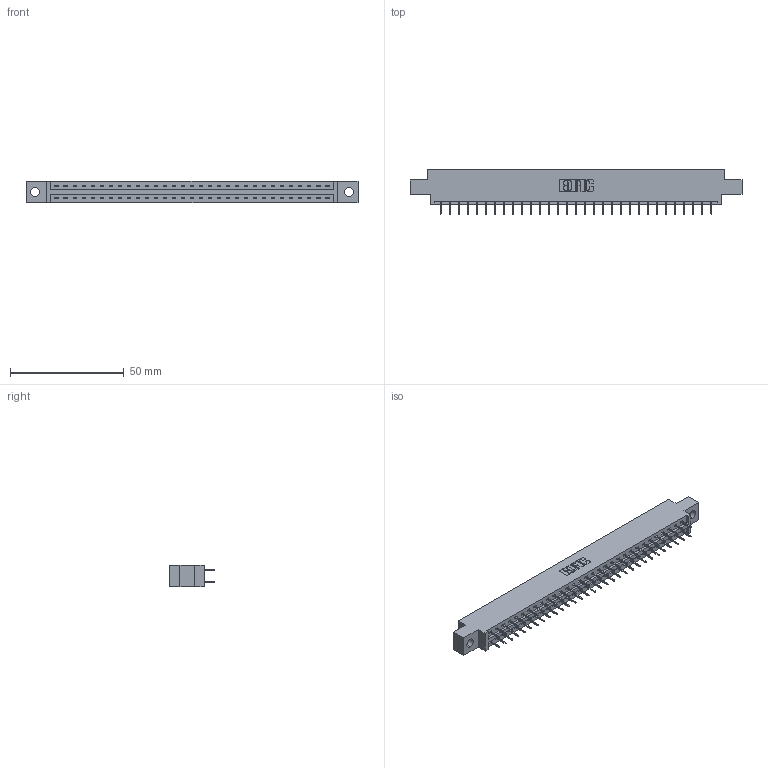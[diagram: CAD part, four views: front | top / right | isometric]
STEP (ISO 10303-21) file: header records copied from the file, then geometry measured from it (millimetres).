
FILE_DESCRIPTION (( 'STEP AP203' ), '1' );
FILE_NAME ('387-062-524-804.STEP', '2019-10-19T14:53:10', ( '' ), ( '' ), 'SwSTEP 2.0', 'SolidWorks 2016', '' );
FILE_SCHEMA (( 'CONFIG_CONTROL_DESIGN' ));
Length unit declared in the file: inch
Products named in the file (3): 345-292-001_345-293-124; 387-062-524-804; 337 Part_0.170 Offset - 0.156 Dia-TH
Assembly tree (63 placements, depth 2):
  387-062-524-804
    337 Part_0.170 Offset - 0.156 Dia-TH
    345-292-001_345-293-124  x62
Bounding box: 145.85 x 19.69 x 9.4 mm (x, y, z)
Volume: 14924.9 mm3; surface area: 16380.4 mm2
Topology: 63 solids, 63 shells, 3714 faces, 10553 edges, 6786 vertices
Faces by surface type: plane 2802, cylinder 912
Entity records: 25667 total; most frequent: CARTESIAN_POINT 4334, ORIENTED_EDGE 4270, DIRECTION 3707, EDGE_CURVE 2135, LINE 2011, VECTOR 2011, VERTEX_POINT 1418, AXIS2_PLACEMENT_3D 848
